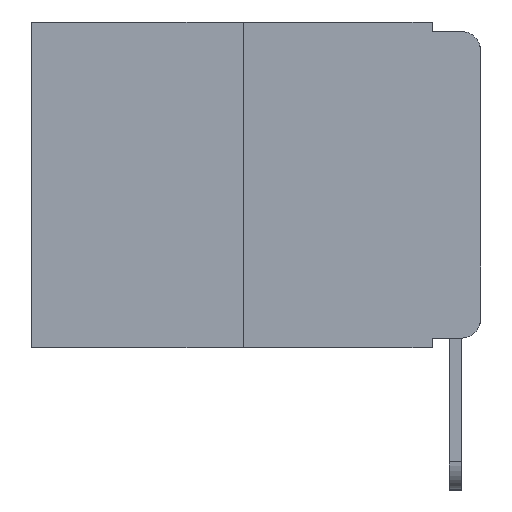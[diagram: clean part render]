
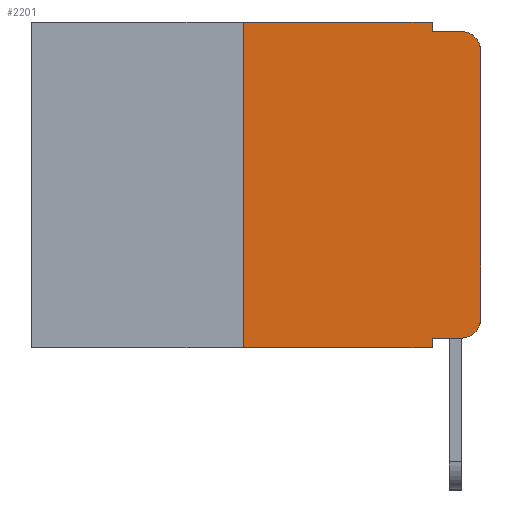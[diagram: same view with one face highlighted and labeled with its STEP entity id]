
A CAD part, left-side view. The second image highlights one B-rep face of the part: STEP entity #2201.
In plain terms, the highlighted planar face has unit normal (-1, 0, 0).
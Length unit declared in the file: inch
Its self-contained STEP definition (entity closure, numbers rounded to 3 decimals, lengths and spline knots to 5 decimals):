
#261 = CARTESIAN_POINT ( 'NONE',  ( 0., 0.25, 0. ) ) ;
#511 = CARTESIAN_POINT ( 'NONE',  ( 0., 0.473, 0. ) ) ;
#602 = CARTESIAN_POINT ( 'NONE',  ( 0., 0.051, 0. ) ) ;
#617 = EDGE_CURVE ( 'NONE', #19186, #14870, #14010, .T. ) ;
#914 = ORIENTED_EDGE ( 'NONE', *, *, #1439, .T. ) ;
#1071 = VECTOR ( 'NONE', #2512, 39.37008 ) ;
#1095 = CARTESIAN_POINT ( 'NONE',  ( 0., 0., -0.313 ) ) ;
#1439 = EDGE_CURVE ( 'NONE', #19842, #19186, #8346, .T. ) ;
#1463 = FACE_OUTER_BOUND ( 'NONE', #6746, .T. ) ;
#1828 = CARTESIAN_POINT ( 'NONE',  ( 0., 0.051, 0. ) ) ;
#2201 = ADVANCED_FACE ( 'NONE', ( #1463 ), #14375, .F. ) ;
#2264 = VERTEX_POINT ( 'NONE', #9600 ) ;
#2277 = LINE ( 'NONE', #3067, #16365 ) ;
#2373 = LINE ( 'NONE', #16502, #11010 ) ;
#2512 = DIRECTION ( 'NONE',  ( 0., 0., -1. ) ) ;
#2863 = VERTEX_POINT ( 'NONE', #1828 ) ;
#3067 = CARTESIAN_POINT ( 'NONE',  ( 0., 0.051, -0.01 ) ) ;
#5180 = ORIENTED_EDGE ( 'NONE', *, *, #14042, .T. ) ;
#6263 = ORIENTED_EDGE ( 'NONE', *, *, #617, .T. ) ;
#6376 = CARTESIAN_POINT ( 'NONE',  ( 0., 0.02, -0.03 ) ) ;
#6744 = DIRECTION ( 'NONE',  ( 0., 0., -1. ) ) ;
#6746 = EDGE_LOOP ( 'NONE', ( #17174, #21879, #14523, #21146, #16928, #15135, #5180, #12088, #914, #6263 ) ) ;
#6923 = CARTESIAN_POINT ( 'NONE',  ( 0., 0.051, -0.01 ) ) ;
#7247 = CARTESIAN_POINT ( 'NONE',  ( 0., 0.02, -0.333 ) ) ;
#7643 = DIRECTION ( 'NONE',  ( 1., 0., 0. ) ) ;
#7830 = VERTEX_POINT ( 'NONE', #21520 ) ;
#8082 = DIRECTION ( 'NONE',  ( 0., 0., -1. ) ) ;
#8346 = LINE ( 'NONE', #20147, #17247 ) ;
#8530 = DIRECTION ( 'NONE',  ( 0., 0., -1. ) ) ;
#8681 = LINE ( 'NONE', #12209, #17035 ) ;
#8785 = AXIS2_PLACEMENT_3D ( 'NONE', #6376, #18097, #8082 ) ;
#8807 = CARTESIAN_POINT ( 'NONE',  ( 0., 0.051, -0.333 ) ) ;
#8913 = VERTEX_POINT ( 'NONE', #6923 ) ;
#9600 = CARTESIAN_POINT ( 'NONE',  ( 0., 0.051, -0.343 ) ) ;
#10394 = LINE ( 'NONE', #602, #1071 ) ;
#11010 = VECTOR ( 'NONE', #18153, 39.37008 ) ;
#11141 = CARTESIAN_POINT ( 'NONE',  ( 0., 0.25, 0. ) ) ;
#11212 = CARTESIAN_POINT ( 'NONE',  ( 0., 0.02, -0.01 ) ) ;
#11403 = EDGE_CURVE ( 'NONE', #8913, #15969, #2277, .T. ) ;
#11592 = DIRECTION ( 'NONE',  ( 0., -1., 0. ) ) ;
#11681 = VECTOR ( 'NONE', #12807, 39.37008 ) ;
#12088 = ORIENTED_EDGE ( 'NONE', *, *, #16637, .F. ) ;
#12209 = CARTESIAN_POINT ( 'NONE',  ( 0., 0., 0. ) ) ;
#12519 = EDGE_CURVE ( 'NONE', #15122, #15969, #21377, .T. ) ;
#12599 = LINE ( 'NONE', #15161, #20777 ) ;
#12797 = CARTESIAN_POINT ( 'NONE',  ( 0., 0.473, -0.343 ) ) ;
#12807 = DIRECTION ( 'NONE',  ( 0., 0., 1. ) ) ;
#12951 = AXIS2_PLACEMENT_3D ( 'NONE', #18183, #20343, #8530 ) ;
#13858 = DIRECTION ( 'NONE',  ( 0., 0., 1. ) ) ;
#14010 = CIRCLE ( 'NONE', #12951, 0.02 ) ;
#14042 = EDGE_CURVE ( 'NONE', #7830, #2264, #21887, .T. ) ;
#14375 = PLANE ( 'NONE',  #20699 ) ;
#14523 = ORIENTED_EDGE ( 'NONE', *, *, #11403, .F. ) ;
#14870 = VERTEX_POINT ( 'NONE', #1095 ) ;
#14935 = DIRECTION ( 'NONE',  ( 0., -1., 0. ) ) ;
#15122 = VERTEX_POINT ( 'NONE', #18663 ) ;
#15135 = ORIENTED_EDGE ( 'NONE', *, *, #17346, .F. ) ;
#15161 = CARTESIAN_POINT ( 'NONE',  ( 0., 0.051, 0. ) ) ;
#15969 = VERTEX_POINT ( 'NONE', #11212 ) ;
#16365 = VECTOR ( 'NONE', #14935, 39.37008 ) ;
#16495 = VERTEX_POINT ( 'NONE', #261 ) ;
#16502 = CARTESIAN_POINT ( 'NONE',  ( 0., 0.473, 0. ) ) ;
#16637 = EDGE_CURVE ( 'NONE', #19842, #2264, #10394, .T. ) ;
#16928 = ORIENTED_EDGE ( 'NONE', *, *, #21183, .F. ) ;
#17035 = VECTOR ( 'NONE', #13858, 39.37008 ) ;
#17174 = ORIENTED_EDGE ( 'NONE', *, *, #18437, .T. ) ;
#17247 = VECTOR ( 'NONE', #11592, 39.37008 ) ;
#17346 = EDGE_CURVE ( 'NONE', #7830, #16495, #20400, .T. ) ;
#17599 = VECTOR ( 'NONE', #21009, 39.37008 ) ;
#18097 = DIRECTION ( 'NONE',  ( -1., 0., 0. ) ) ;
#18153 = DIRECTION ( 'NONE',  ( 0., -1., 0. ) ) ;
#18183 = CARTESIAN_POINT ( 'NONE',  ( 0., 0.02, -0.313 ) ) ;
#18437 = EDGE_CURVE ( 'NONE', #14870, #15122, #8681, .T. ) ;
#18663 = CARTESIAN_POINT ( 'NONE',  ( 0., 0., -0.03 ) ) ;
#19186 = VERTEX_POINT ( 'NONE', #7247 ) ;
#19318 = DIRECTION ( 'NONE',  ( 0., 0., -1. ) ) ;
#19842 = VERTEX_POINT ( 'NONE', #8807 ) ;
#20147 = CARTESIAN_POINT ( 'NONE',  ( 0., 0.051, -0.333 ) ) ;
#20343 = DIRECTION ( 'NONE',  ( -1., 0., 0. ) ) ;
#20400 = LINE ( 'NONE', #11141, #11681 ) ;
#20606 = EDGE_CURVE ( 'NONE', #2863, #8913, #12599, .T. ) ;
#20699 = AXIS2_PLACEMENT_3D ( 'NONE', #511, #7643, #19318 ) ;
#20777 = VECTOR ( 'NONE', #6744, 39.37008 ) ;
#21009 = DIRECTION ( 'NONE',  ( 0., -1., 0. ) ) ;
#21146 = ORIENTED_EDGE ( 'NONE', *, *, #20606, .F. ) ;
#21183 = EDGE_CURVE ( 'NONE', #16495, #2863, #2373, .T. ) ;
#21377 = CIRCLE ( 'NONE', #8785, 0.02 ) ;
#21520 = CARTESIAN_POINT ( 'NONE',  ( 0., 0.25, -0.343 ) ) ;
#21879 = ORIENTED_EDGE ( 'NONE', *, *, #12519, .T. ) ;
#21887 = LINE ( 'NONE', #12797, #17599 ) ;
